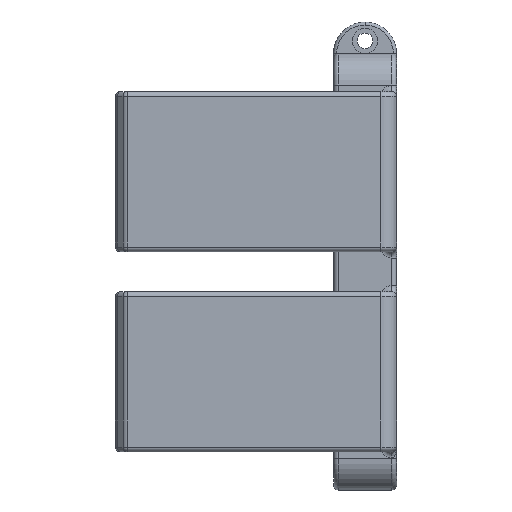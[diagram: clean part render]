
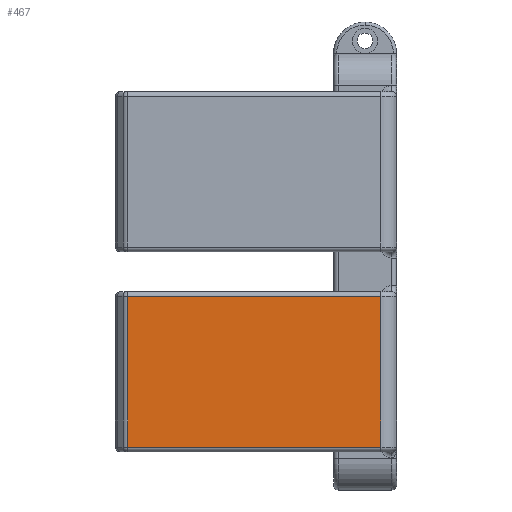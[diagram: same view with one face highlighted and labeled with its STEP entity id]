
A CAD part, left-side view. The second image highlights one B-rep face of the part: STEP entity #467.
In plain terms, the highlighted planar face has unit normal (-1, 0, 0).
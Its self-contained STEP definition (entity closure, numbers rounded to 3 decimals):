
#93 = PLANE ( 'NONE',  #1153 ) ;
#330 = FACE_OUTER_BOUND ( 'NONE', #4085, .T. ) ;
#384 = VECTOR ( 'NONE', #474, 1000. ) ;
#413 = ORIENTED_EDGE ( 'NONE', *, *, #3515, .T. ) ;
#467 = ADVANCED_FACE ( 'NONE', ( #330 ), #93, .T. ) ;
#474 = DIRECTION ( 'NONE',  ( 0., 0., -1. ) ) ;
#549 = DIRECTION ( 'NONE',  ( -1., 0., 0. ) ) ;
#677 = EDGE_CURVE ( 'NONE', #3277, #3049, #2706, .T. ) ;
#923 = CARTESIAN_POINT ( 'NONE',  ( -18.312, 48.07, 0. ) ) ;
#1152 = ORIENTED_EDGE ( 'NONE', *, *, #1389, .T. ) ;
#1153 = AXIS2_PLACEMENT_3D ( 'NONE', #4102, #549, #3682 ) ;
#1267 = DIRECTION ( 'NONE',  ( 0., 1., 0. ) ) ;
#1277 = EDGE_CURVE ( 'NONE', #3049, #4213, #5600, .T. ) ;
#1389 = EDGE_CURVE ( 'NONE', #5361, #3277, #1584, .T. ) ;
#1584 = LINE ( 'NONE', #923, #384 ) ;
#1748 = CARTESIAN_POINT ( 'NONE',  ( -18.312, 48.07, -27.825 ) ) ;
#1868 = DIRECTION ( 'NONE',  ( 0., 0., 1. ) ) ;
#2448 = VECTOR ( 'NONE', #4312, 1000. ) ;
#2555 = CARTESIAN_POINT ( 'NONE',  ( -18.312, 7.884, -27.825 ) ) ;
#2706 = LINE ( 'NONE', #2555, #2448 ) ;
#2709 = CARTESIAN_POINT ( 'NONE',  ( -18.312, 7.884, -27.825 ) ) ;
#3049 = VERTEX_POINT ( 'NONE', #2709 ) ;
#3277 = VERTEX_POINT ( 'NONE', #1748 ) ;
#3515 = EDGE_CURVE ( 'NONE', #4213, #5361, #3794, .T. ) ;
#3647 = VECTOR ( 'NONE', #1267, 1000. ) ;
#3682 = DIRECTION ( 'NONE',  ( 0., 0., 1. ) ) ;
#3794 = LINE ( 'NONE', #3934, #3647 ) ;
#3825 = ORIENTED_EDGE ( 'NONE', *, *, #1277, .T. ) ;
#3934 = CARTESIAN_POINT ( 'NONE',  ( -18.312, 48.07, -3.925 ) ) ;
#4085 = EDGE_LOOP ( 'NONE', ( #1152, #5405, #3825, #413 ) ) ;
#4102 = CARTESIAN_POINT ( 'NONE',  ( -18.312, 0., 0. ) ) ;
#4213 = VERTEX_POINT ( 'NONE', #4573 ) ;
#4312 = DIRECTION ( 'NONE',  ( 0., -1., 0. ) ) ;
#4491 = VECTOR ( 'NONE', #1868, 1000. ) ;
#4503 = CARTESIAN_POINT ( 'NONE',  ( -18.312, 7.884, -3.175 ) ) ;
#4573 = CARTESIAN_POINT ( 'NONE',  ( -18.312, 7.884, -3.925 ) ) ;
#5312 = CARTESIAN_POINT ( 'NONE',  ( -18.312, 48.07, -3.925 ) ) ;
#5361 = VERTEX_POINT ( 'NONE', #5312 ) ;
#5405 = ORIENTED_EDGE ( 'NONE', *, *, #677, .T. ) ;
#5600 = LINE ( 'NONE', #4503, #4491 ) ;
